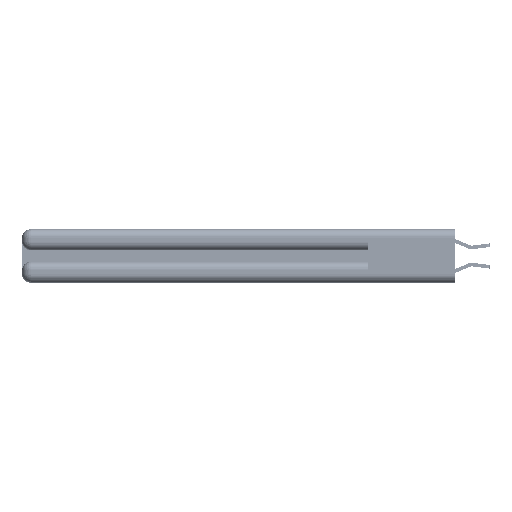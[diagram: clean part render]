
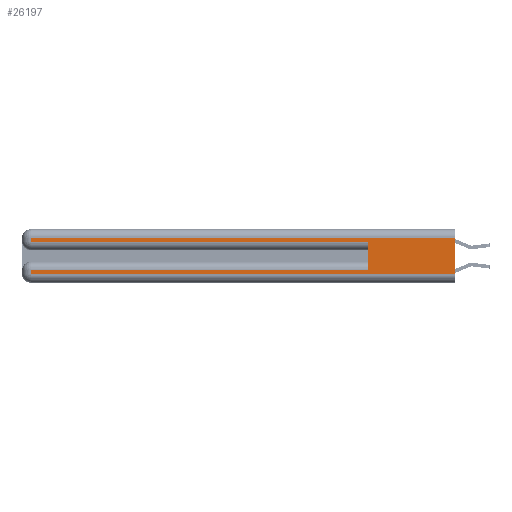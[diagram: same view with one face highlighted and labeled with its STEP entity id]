
A CAD part, left-side view. The second image highlights one B-rep face of the part: STEP entity #26197.
In plain terms, the highlighted planar face has unit normal (-1, 0, 0).
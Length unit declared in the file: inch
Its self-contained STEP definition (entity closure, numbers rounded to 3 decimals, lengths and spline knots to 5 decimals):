
#1036 = VECTOR ( 'NONE', #12042, 39.37008 ) ;
#1307 = VERTEX_POINT ( 'NONE', #15114 ) ;
#1666 = VECTOR ( 'NONE', #27257, 39.37008 ) ;
#3249 = DIRECTION ( 'NONE',  ( 0., 0., -1. ) ) ;
#4515 = CARTESIAN_POINT ( 'NONE',  ( 0., 0., 0.37 ) ) ;
#4850 = LINE ( 'NONE', #16781, #17319 ) ;
#5408 = CARTESIAN_POINT ( 'NONE',  ( 0., 0., 0.31 ) ) ;
#5766 = VERTEX_POINT ( 'NONE', #25525 ) ;
#5791 = EDGE_LOOP ( 'NONE', ( #17305, #27890, #13677, #27414, #11718, #12263, #25306, #11997 ) ) ;
#6284 = EDGE_CURVE ( 'NONE', #15604, #34425, #12844, .T. ) ;
#7061 = VECTOR ( 'NONE', #23362, 39.37008 ) ;
#7096 = VECTOR ( 'NONE', #34590, 39.37008 ) ;
#7198 = PLANE ( 'NONE',  #26870 ) ;
#7236 = EDGE_CURVE ( 'NONE', #25602, #5766, #14905, .T. ) ;
#9503 = LINE ( 'NONE', #32233, #30028 ) ;
#10543 = CARTESIAN_POINT ( 'NONE',  ( 0., 0., 0.085 ) ) ;
#11194 = CARTESIAN_POINT ( 'NONE',  ( 0., 2.94, 0.37 ) ) ;
#11472 = EDGE_CURVE ( 'NONE', #14094, #1307, #13771, .T. ) ;
#11540 = CARTESIAN_POINT ( 'NONE',  ( 0., 0.6, 0.085 ) ) ;
#11718 = ORIENTED_EDGE ( 'NONE', *, *, #7236, .F. ) ;
#11872 = CARTESIAN_POINT ( 'NONE',  ( 0., 2.94, 0.285 ) ) ;
#11997 = ORIENTED_EDGE ( 'NONE', *, *, #11472, .T. ) ;
#12042 = DIRECTION ( 'NONE',  ( 0., 0., -1. ) ) ;
#12149 = DIRECTION ( 'NONE',  ( 0., 0., 1. ) ) ;
#12263 = ORIENTED_EDGE ( 'NONE', *, *, #32120, .T. ) ;
#12844 = LINE ( 'NONE', #11194, #7061 ) ;
#13247 = VERTEX_POINT ( 'NONE', #5408 ) ;
#13677 = ORIENTED_EDGE ( 'NONE', *, *, #6284, .T. ) ;
#13771 = LINE ( 'NONE', #14427, #7096 ) ;
#14094 = VERTEX_POINT ( 'NONE', #31391 ) ;
#14427 = CARTESIAN_POINT ( 'NONE',  ( 0., 0., 0.06 ) ) ;
#14905 = LINE ( 'NONE', #23587, #29207 ) ;
#15114 = CARTESIAN_POINT ( 'NONE',  ( 0., 0., 0.06 ) ) ;
#15604 = VERTEX_POINT ( 'NONE', #22537 ) ;
#16781 = CARTESIAN_POINT ( 'NONE',  ( 0., 0., 0.285 ) ) ;
#16904 = DIRECTION ( 'NONE',  ( 0., -1., 0. ) ) ;
#17305 = ORIENTED_EDGE ( 'NONE', *, *, #26481, .F. ) ;
#17319 = VECTOR ( 'NONE', #16904, 39.37008 ) ;
#18488 = DIRECTION ( 'NONE',  ( 0., 0., -1. ) ) ;
#20148 = VERTEX_POINT ( 'NONE', #24265 ) ;
#21474 = DIRECTION ( 'NONE',  ( 0., 1., 0. ) ) ;
#22537 = CARTESIAN_POINT ( 'NONE',  ( 0., 2.94, 0.31 ) ) ;
#22588 = EDGE_CURVE ( 'NONE', #13247, #15604, #25336, .T. ) ;
#22769 = LINE ( 'NONE', #10543, #28160 ) ;
#23362 = DIRECTION ( 'NONE',  ( 0., 0., -1. ) ) ;
#23488 = CARTESIAN_POINT ( 'NONE',  ( 0., 2.94, 0.37 ) ) ;
#23587 = CARTESIAN_POINT ( 'NONE',  ( 0., 0.6, 0.145 ) ) ;
#24265 = CARTESIAN_POINT ( 'NONE',  ( 0., 2.94, 0.085 ) ) ;
#24487 = DIRECTION ( 'NONE',  ( 1., 0., 0. ) ) ;
#25306 = ORIENTED_EDGE ( 'NONE', *, *, #29070, .T. ) ;
#25336 = LINE ( 'NONE', #27373, #1666 ) ;
#25525 = CARTESIAN_POINT ( 'NONE',  ( 0., 0.6, 0.285 ) ) ;
#25602 = VERTEX_POINT ( 'NONE', #11540 ) ;
#26197 = ADVANCED_FACE ( 'NONE', ( #30452 ), #7198, .F. ) ;
#26481 = EDGE_CURVE ( 'NONE', #13247, #1307, #9503, .T. ) ;
#26870 = AXIS2_PLACEMENT_3D ( 'NONE', #4515, #24487, #18488 ) ;
#27257 = DIRECTION ( 'NONE',  ( 0., 1., 0. ) ) ;
#27373 = CARTESIAN_POINT ( 'NONE',  ( 0., 0., 0.31 ) ) ;
#27414 = ORIENTED_EDGE ( 'NONE', *, *, #32977, .T. ) ;
#27890 = ORIENTED_EDGE ( 'NONE', *, *, #22588, .T. ) ;
#28160 = VECTOR ( 'NONE', #21474, 39.37008 ) ;
#29070 = EDGE_CURVE ( 'NONE', #20148, #14094, #33715, .T. ) ;
#29207 = VECTOR ( 'NONE', #12149, 39.37008 ) ;
#30028 = VECTOR ( 'NONE', #3249, 39.37008 ) ;
#30452 = FACE_OUTER_BOUND ( 'NONE', #5791, .T. ) ;
#31391 = CARTESIAN_POINT ( 'NONE',  ( 0., 2.94, 0.06 ) ) ;
#32120 = EDGE_CURVE ( 'NONE', #25602, #20148, #22769, .T. ) ;
#32233 = CARTESIAN_POINT ( 'NONE',  ( 0., 0., 0.37 ) ) ;
#32977 = EDGE_CURVE ( 'NONE', #34425, #5766, #4850, .T. ) ;
#33715 = LINE ( 'NONE', #23488, #1036 ) ;
#34425 = VERTEX_POINT ( 'NONE', #11872 ) ;
#34590 = DIRECTION ( 'NONE',  ( 0., -1., 0. ) ) ;
